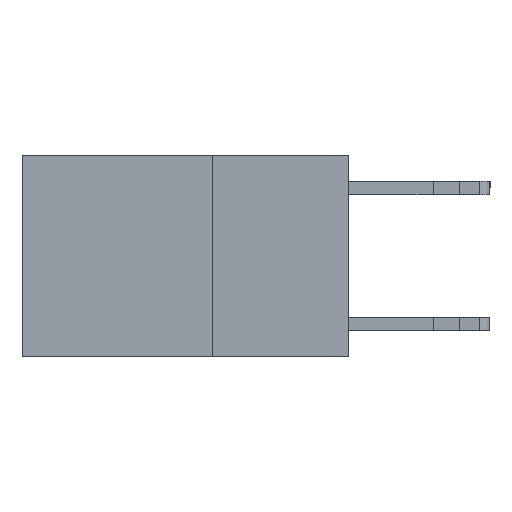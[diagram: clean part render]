
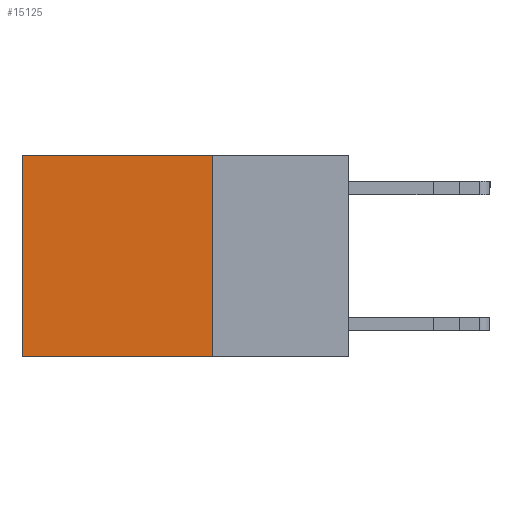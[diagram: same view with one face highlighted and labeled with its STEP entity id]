
A CAD part, left-side view. The second image highlights one B-rep face of the part: STEP entity #15125.
In plain terms, the highlighted planar face has unit normal (-1, 0, 0).
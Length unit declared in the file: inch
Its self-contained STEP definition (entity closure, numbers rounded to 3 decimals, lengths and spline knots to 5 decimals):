
#426 = ORIENTED_EDGE ( 'NONE', *, *, #18046, .F. ) ;
#536 = CARTESIAN_POINT ( 'NONE',  ( 0.2625, 0.25, 0. ) ) ;
#1581 = CARTESIAN_POINT ( 'NONE',  ( 0.2625, 0.25, -0.37 ) ) ;
#2109 = LINE ( 'NONE', #536, #10167 ) ;
#2729 = ORIENTED_EDGE ( 'NONE', *, *, #20165, .T. ) ;
#3002 = DIRECTION ( 'NONE',  ( 0., 0., -1. ) ) ;
#3986 = CARTESIAN_POINT ( 'NONE',  ( 0.2625, 0.25, 0. ) ) ;
#4123 = CARTESIAN_POINT ( 'NONE',  ( 0.2625, 0.6, -0.37 ) ) ;
#4511 = EDGE_CURVE ( 'NONE', #13355, #18838, #18621, .T. ) ;
#4532 = VECTOR ( 'NONE', #5263, 39.37008 ) ;
#4648 = CARTESIAN_POINT ( 'NONE',  ( 0.2625, 0.25, -0.37 ) ) ;
#5263 = DIRECTION ( 'NONE',  ( 0., 0., -1. ) ) ;
#5270 = VECTOR ( 'NONE', #8017, 39.37008 ) ;
#5879 = LINE ( 'NONE', #3986, #5270 ) ;
#5949 = EDGE_CURVE ( 'NONE', #9673, #18838, #9762, .T. ) ;
#6864 = DIRECTION ( 'NONE',  ( 0., 1., 0. ) ) ;
#8017 = DIRECTION ( 'NONE',  ( 0., 0., -1. ) ) ;
#9277 = VERTEX_POINT ( 'NONE', #11322 ) ;
#9673 = VERTEX_POINT ( 'NONE', #9979 ) ;
#9749 = AXIS2_PLACEMENT_3D ( 'NONE', #19791, #10390, #3002 ) ;
#9762 = LINE ( 'NONE', #9855, #4532 ) ;
#9855 = CARTESIAN_POINT ( 'NONE',  ( 0.2625, 0.6, 0. ) ) ;
#9979 = CARTESIAN_POINT ( 'NONE',  ( 0.2625, 0.6, 0. ) ) ;
#10167 = VECTOR ( 'NONE', #6864, 39.37008 ) ;
#10390 = DIRECTION ( 'NONE',  ( 1., 0., 0. ) ) ;
#10883 = DIRECTION ( 'NONE',  ( 0., 1., 0. ) ) ;
#11322 = CARTESIAN_POINT ( 'NONE',  ( 0.2625, 0.25, 0. ) ) ;
#13355 = VERTEX_POINT ( 'NONE', #1581 ) ;
#14780 = ORIENTED_EDGE ( 'NONE', *, *, #5949, .T. ) ;
#15125 = ADVANCED_FACE ( 'NONE', ( #15386 ), #16898, .F. ) ;
#15386 = FACE_OUTER_BOUND ( 'NONE', #15499, .T. ) ;
#15499 = EDGE_LOOP ( 'NONE', ( #14780, #18472, #426, #2729 ) ) ;
#16792 = VECTOR ( 'NONE', #10883, 39.37008 ) ;
#16898 = PLANE ( 'NONE',  #9749 ) ;
#18046 = EDGE_CURVE ( 'NONE', #9277, #13355, #5879, .T. ) ;
#18472 = ORIENTED_EDGE ( 'NONE', *, *, #4511, .F. ) ;
#18621 = LINE ( 'NONE', #4648, #16792 ) ;
#18838 = VERTEX_POINT ( 'NONE', #4123 ) ;
#19791 = CARTESIAN_POINT ( 'NONE',  ( 0.2625, 0.25, 0. ) ) ;
#20165 = EDGE_CURVE ( 'NONE', #9277, #9673, #2109, .T. ) ;
